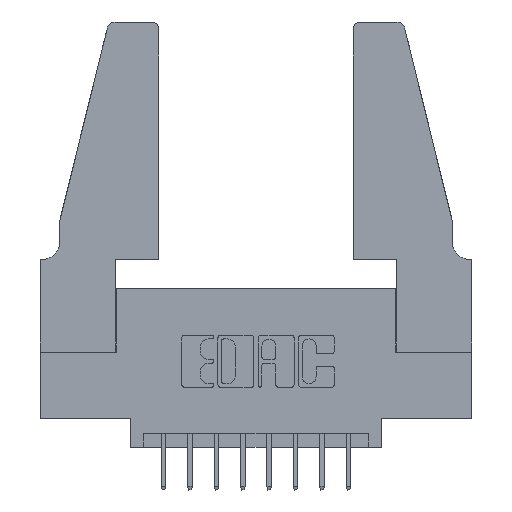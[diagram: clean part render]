
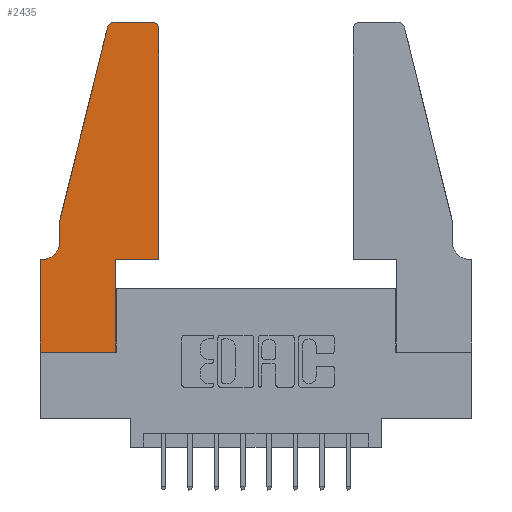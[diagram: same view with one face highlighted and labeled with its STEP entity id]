
A CAD part, top view. The second image highlights one B-rep face of the part: STEP entity #2435.
In plain terms, the highlighted planar face has unit normal (0, 0, 1).
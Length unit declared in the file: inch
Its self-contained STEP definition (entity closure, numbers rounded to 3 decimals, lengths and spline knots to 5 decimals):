
#131 = VERTEX_POINT ( 'NONE', #10086 ) ;
#343 = ORIENTED_EDGE ( 'NONE', *, *, #7341, .T. ) ;
#431 = VERTEX_POINT ( 'NONE', #2654 ) ;
#439 = DIRECTION ( 'NONE',  ( 0., -1., 0. ) ) ;
#480 = CARTESIAN_POINT ( 'NONE',  ( 0.4505, 0.35, 0.37 ) ) ;
#680 = CIRCLE ( 'NONE', #5142, 0.03 ) ;
#767 = VECTOR ( 'NONE', #9067, 39.37008 ) ;
#800 = DIRECTION ( 'NONE',  ( -1., 0., 0. ) ) ;
#878 = CARTESIAN_POINT ( 'NONE',  ( 0.4505, 0.35, 0.37 ) ) ;
#953 = DIRECTION ( 'NONE',  ( 0., 1., 0. ) ) ;
#993 = ORIENTED_EDGE ( 'NONE', *, *, #8176, .T. ) ;
#1025 = VECTOR ( 'NONE', #11970, 39.37008 ) ;
#1088 = VERTEX_POINT ( 'NONE', #5850 ) ;
#1170 = VECTOR ( 'NONE', #1992, 39.37008 ) ;
#1176 = CARTESIAN_POINT ( 'NONE',  ( 0., 0., 0.37 ) ) ;
#1383 = VERTEX_POINT ( 'NONE', #2068 ) ;
#1535 = VERTEX_POINT ( 'NONE', #8510 ) ;
#1923 = EDGE_CURVE ( 'NONE', #10936, #1383, #3908, .T. ) ;
#1992 = DIRECTION ( 'NONE',  ( 0., 1., 0. ) ) ;
#2068 = CARTESIAN_POINT ( 'NONE',  ( 0.0755, 0.5, 0.37 ) ) ;
#2435 = ADVANCED_FACE ( 'NONE', ( #9000 ), #8994, .T. ) ;
#2438 = VECTOR ( 'NONE', #13148, 39.37008 ) ;
#2469 = EDGE_CURVE ( 'NONE', #431, #10936, #680, .T. ) ;
#2654 = CARTESIAN_POINT ( 'NONE',  ( 0.284, 1.25, 0.37 ) ) ;
#2706 = VECTOR ( 'NONE', #800, 39.37008 ) ;
#3367 = AXIS2_PLACEMENT_3D ( 'NONE', #10923, #4878, #11910 ) ;
#3908 = LINE ( 'NONE', #7414, #1025 ) ;
#3988 = CARTESIAN_POINT ( 'NONE',  ( 0.4205, 1.25, 0.37 ) ) ;
#3990 = CARTESIAN_POINT ( 'NONE',  ( 0.4505, 0.35, 0.37 ) ) ;
#4228 = CARTESIAN_POINT ( 'NONE',  ( 0.0055, 0.42, 0.37 ) ) ;
#4364 = CIRCLE ( 'NONE', #3367, 0.03 ) ;
#4428 = VERTEX_POINT ( 'NONE', #1176 ) ;
#4446 = AXIS2_PLACEMENT_3D ( 'NONE', #8769, #8632, #8619 ) ;
#4589 = ORIENTED_EDGE ( 'NONE', *, *, #1923, .T. ) ;
#4847 = CARTESIAN_POINT ( 'NONE',  ( 0.2865, 0., 0.37 ) ) ;
#4878 = DIRECTION ( 'NONE',  ( 0., 0., 1. ) ) ;
#5121 = AXIS2_PLACEMENT_3D ( 'NONE', #4228, #11283, #5275 ) ;
#5142 = AXIS2_PLACEMENT_3D ( 'NONE', #8127, #8115, #8086 ) ;
#5167 = CARTESIAN_POINT ( 'NONE',  ( 0.0755, 0.5, 0.37 ) ) ;
#5219 = DIRECTION ( 'NONE',  ( -1., 0., 0. ) ) ;
#5275 = DIRECTION ( 'NONE',  ( -1., 0., 0. ) ) ;
#5327 = VERTEX_POINT ( 'NONE', #5825 ) ;
#5451 = EDGE_CURVE ( 'NONE', #4428, #9002, #8754, .T. ) ;
#5504 = ORIENTED_EDGE ( 'NONE', *, *, #5451, .T. ) ;
#5638 = ORIENTED_EDGE ( 'NONE', *, *, #11403, .T. ) ;
#5825 = CARTESIAN_POINT ( 'NONE',  ( 0.0055, 0.35, 0.37 ) ) ;
#5850 = CARTESIAN_POINT ( 'NONE',  ( 0.4505, 1.22, 0.37 ) ) ;
#5875 = LINE ( 'NONE', #5167, #2438 ) ;
#6248 = CARTESIAN_POINT ( 'NONE',  ( 0.0755, 0.35, 0.37 ) ) ;
#6294 = ORIENTED_EDGE ( 'NONE', *, *, #11522, .T. ) ;
#6363 = EDGE_CURVE ( 'NONE', #5327, #131, #9568, .T. ) ;
#6443 = CIRCLE ( 'NONE', #5121, 0.07 ) ;
#6760 = LINE ( 'NONE', #878, #1170 ) ;
#6998 = EDGE_LOOP ( 'NONE', ( #6294, #9469, #4589, #11558, #8723, #12983, #343, #5504, #8046, #993, #8091, #5638 ) ) ;
#7244 = CARTESIAN_POINT ( 'NONE',  ( 0.2865, 0.35, 0.37 ) ) ;
#7341 = EDGE_CURVE ( 'NONE', #131, #4428, #10309, .T. ) ;
#7414 = CARTESIAN_POINT ( 'NONE',  ( 0.0755, 0.5, 0.37 ) ) ;
#7640 = VECTOR ( 'NONE', #439, 39.37008 ) ;
#8027 = CARTESIAN_POINT ( 'NONE',  ( 0., 0., 0.37 ) ) ;
#8046 = ORIENTED_EDGE ( 'NONE', *, *, #10970, .T. ) ;
#8086 = DIRECTION ( 'NONE',  ( 1., 0., 0. ) ) ;
#8091 = ORIENTED_EDGE ( 'NONE', *, *, #10327, .T. ) ;
#8115 = DIRECTION ( 'NONE',  ( 0., 0., 1. ) ) ;
#8127 = CARTESIAN_POINT ( 'NONE',  ( 0.284, 1.22, 0.37 ) ) ;
#8158 = LINE ( 'NONE', #11131, #2706 ) ;
#8176 = EDGE_CURVE ( 'NONE', #8977, #10075, #8887, .T. ) ;
#8282 = EDGE_CURVE ( 'NONE', #1383, #1535, #5875, .T. ) ;
#8510 = CARTESIAN_POINT ( 'NONE',  ( 0.0755, 0.42, 0.37 ) ) ;
#8619 = DIRECTION ( 'NONE',  ( 1., 0., 0. ) ) ;
#8632 = DIRECTION ( 'NONE',  ( 0., 0., 1. ) ) ;
#8723 = ORIENTED_EDGE ( 'NONE', *, *, #10351, .T. ) ;
#8730 = CARTESIAN_POINT ( 'NONE',  ( 0., 0., 0.37 ) ) ;
#8754 = LINE ( 'NONE', #8027, #767 ) ;
#8769 = CARTESIAN_POINT ( 'NONE',  ( 0., 0.35, 0.37 ) ) ;
#8887 = LINE ( 'NONE', #3990, #11510 ) ;
#8977 = VERTEX_POINT ( 'NONE', #11414 ) ;
#8994 = PLANE ( 'NONE',  #4446 ) ;
#9000 = FACE_OUTER_BOUND ( 'NONE', #6998, .T. ) ;
#9002 = VERTEX_POINT ( 'NONE', #4847 ) ;
#9067 = DIRECTION ( 'NONE',  ( 1., 0., 0. ) ) ;
#9097 = VERTEX_POINT ( 'NONE', #3988 ) ;
#9469 = ORIENTED_EDGE ( 'NONE', *, *, #2469, .T. ) ;
#9568 = LINE ( 'NONE', #6248, #11554 ) ;
#9599 = LINE ( 'NONE', #7244, #11906 ) ;
#10075 = VERTEX_POINT ( 'NONE', #480 ) ;
#10086 = CARTESIAN_POINT ( 'NONE',  ( 0., 0.35, 0.37 ) ) ;
#10185 = CARTESIAN_POINT ( 'NONE',  ( 0.25487, 1.22718, 0.37 ) ) ;
#10309 = LINE ( 'NONE', #8730, #7640 ) ;
#10327 = EDGE_CURVE ( 'NONE', #10075, #1088, #6760, .T. ) ;
#10351 = EDGE_CURVE ( 'NONE', #1535, #5327, #6443, .T. ) ;
#10923 = CARTESIAN_POINT ( 'NONE',  ( 0.4205, 1.22, 0.37 ) ) ;
#10936 = VERTEX_POINT ( 'NONE', #10185 ) ;
#10970 = EDGE_CURVE ( 'NONE', #9002, #8977, #9599, .T. ) ;
#11131 = CARTESIAN_POINT ( 'NONE',  ( 0.2605, 1.25, 0.37 ) ) ;
#11283 = DIRECTION ( 'NONE',  ( 0., 0., -1. ) ) ;
#11403 = EDGE_CURVE ( 'NONE', #1088, #9097, #4364, .T. ) ;
#11414 = CARTESIAN_POINT ( 'NONE',  ( 0.2865, 0.35, 0.37 ) ) ;
#11510 = VECTOR ( 'NONE', #13020, 39.37008 ) ;
#11522 = EDGE_CURVE ( 'NONE', #9097, #431, #8158, .T. ) ;
#11554 = VECTOR ( 'NONE', #5219, 39.37008 ) ;
#11558 = ORIENTED_EDGE ( 'NONE', *, *, #8282, .T. ) ;
#11906 = VECTOR ( 'NONE', #953, 39.37008 ) ;
#11910 = DIRECTION ( 'NONE',  ( 1., 0., 0. ) ) ;
#11970 = DIRECTION ( 'NONE',  ( -0.239, -0.971, 0. ) ) ;
#12983 = ORIENTED_EDGE ( 'NONE', *, *, #6363, .T. ) ;
#13020 = DIRECTION ( 'NONE',  ( 1., 0., 0. ) ) ;
#13148 = DIRECTION ( 'NONE',  ( 0., -1., 0. ) ) ;
